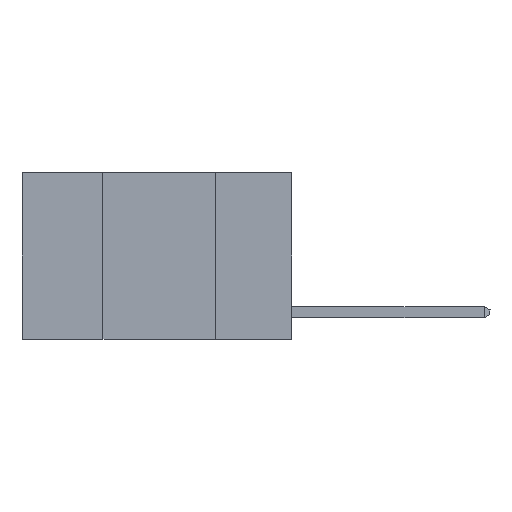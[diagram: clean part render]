
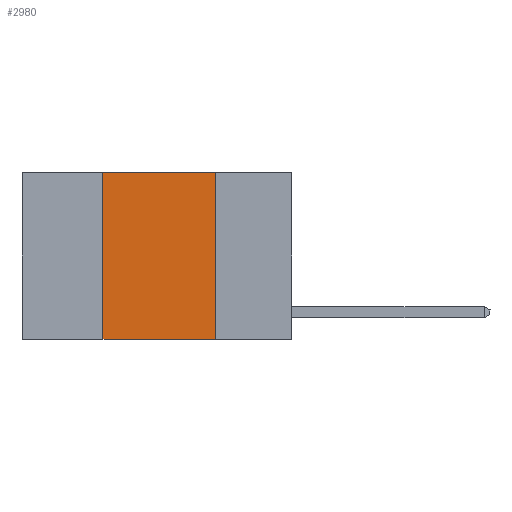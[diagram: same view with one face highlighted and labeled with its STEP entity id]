
A CAD part, left-side view. The second image highlights one B-rep face of the part: STEP entity #2980.
In plain terms, the highlighted planar face has unit normal (-1, 0, 0).
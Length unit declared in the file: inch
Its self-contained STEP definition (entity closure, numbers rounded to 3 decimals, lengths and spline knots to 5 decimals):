
#1125 = CARTESIAN_POINT ( 'NONE',  ( 0., 0.17, 0. ) ) ;
#2025 = VECTOR ( 'NONE', #9803, 39.37008 ) ;
#2403 = DIRECTION ( 'NONE',  ( 1., 0., 0. ) ) ;
#2418 = LINE ( 'NONE', #8635, #2025 ) ;
#2464 = LINE ( 'NONE', #6114, #11122 ) ;
#2980 = ADVANCED_FACE ( 'NONE', ( #14470 ), #11512, .F. ) ;
#4074 = EDGE_CURVE ( 'NONE', #11609, #13139, #10536, .T. ) ;
#4199 = DIRECTION ( 'NONE',  ( 0., 0., 1. ) ) ;
#4370 = DIRECTION ( 'NONE',  ( 0., -1., 0. ) ) ;
#5534 = CARTESIAN_POINT ( 'NONE',  ( 0., 0.17, -0.37 ) ) ;
#6114 = CARTESIAN_POINT ( 'NONE',  ( 0., 0.17, 0. ) ) ;
#6199 = ORIENTED_EDGE ( 'NONE', *, *, #9813, .F. ) ;
#6391 = AXIS2_PLACEMENT_3D ( 'NONE', #14280, #2403, #9258 ) ;
#6483 = EDGE_LOOP ( 'NONE', ( #8684, #14547, #6199, #12035 ) ) ;
#7033 = VERTEX_POINT ( 'NONE', #11912 ) ;
#7204 = DIRECTION ( 'NONE',  ( 0., 0., -1. ) ) ;
#7540 = CARTESIAN_POINT ( 'NONE',  ( 0., 0.42, 0. ) ) ;
#7621 = LINE ( 'NONE', #7540, #10239 ) ;
#8635 = CARTESIAN_POINT ( 'NONE',  ( 0., 0.6, -0.37 ) ) ;
#8684 = ORIENTED_EDGE ( 'NONE', *, *, #9023, .F. ) ;
#9023 = EDGE_CURVE ( 'NONE', #13139, #13718, #2464, .T. ) ;
#9258 = DIRECTION ( 'NONE',  ( 0., 0., -1. ) ) ;
#9803 = DIRECTION ( 'NONE',  ( 0., -1., 0. ) ) ;
#9813 = EDGE_CURVE ( 'NONE', #7033, #11609, #7621, .T. ) ;
#10189 = VECTOR ( 'NONE', #4370, 39.37008 ) ;
#10239 = VECTOR ( 'NONE', #4199, 39.37008 ) ;
#10536 = LINE ( 'NONE', #12151, #10189 ) ;
#10564 = EDGE_CURVE ( 'NONE', #7033, #13718, #2418, .T. ) ;
#11122 = VECTOR ( 'NONE', #7204, 39.37008 ) ;
#11512 = PLANE ( 'NONE',  #6391 ) ;
#11609 = VERTEX_POINT ( 'NONE', #12222 ) ;
#11912 = CARTESIAN_POINT ( 'NONE',  ( 0., 0.42, -0.37 ) ) ;
#12035 = ORIENTED_EDGE ( 'NONE', *, *, #10564, .T. ) ;
#12151 = CARTESIAN_POINT ( 'NONE',  ( 0., 0.6, 0. ) ) ;
#12222 = CARTESIAN_POINT ( 'NONE',  ( 0., 0.42, 0. ) ) ;
#13139 = VERTEX_POINT ( 'NONE', #1125 ) ;
#13718 = VERTEX_POINT ( 'NONE', #5534 ) ;
#14280 = CARTESIAN_POINT ( 'NONE',  ( 0., 0.6, 0. ) ) ;
#14470 = FACE_OUTER_BOUND ( 'NONE', #6483, .T. ) ;
#14547 = ORIENTED_EDGE ( 'NONE', *, *, #4074, .F. ) ;
